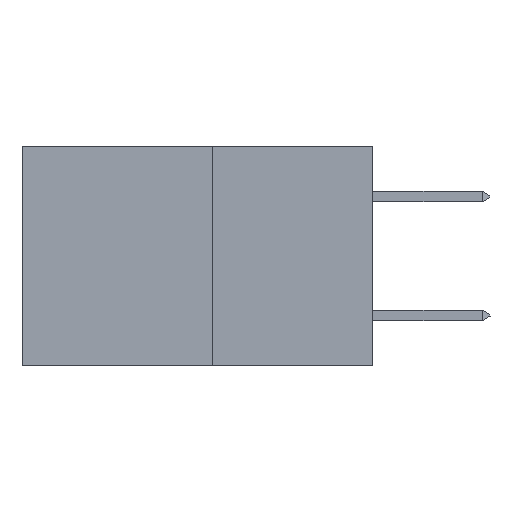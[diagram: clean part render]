
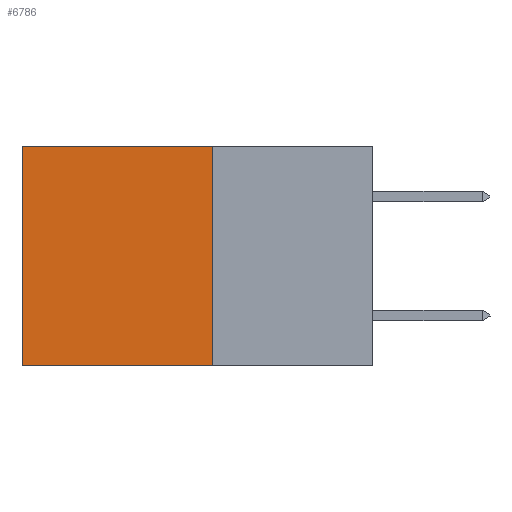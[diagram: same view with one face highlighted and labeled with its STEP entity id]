
A CAD part, left-side view. The second image highlights one B-rep face of the part: STEP entity #6786.
In plain terms, the highlighted planar face has unit normal (-1, 0, 0).
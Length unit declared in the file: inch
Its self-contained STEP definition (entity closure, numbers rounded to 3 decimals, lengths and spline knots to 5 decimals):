
#209 = CARTESIAN_POINT ( 'NONE',  ( 0.277, 0.27, -0.37 ) ) ;
#285 = EDGE_CURVE ( 'NONE', #6105, #10315, #3829, .T. ) ;
#513 = CARTESIAN_POINT ( 'NONE',  ( 0.277, 0.59, 0. ) ) ;
#526 = EDGE_CURVE ( 'NONE', #11175, #8962, #9156, .T. ) ;
#1285 = ORIENTED_EDGE ( 'NONE', *, *, #2825, .T. ) ;
#1349 = ORIENTED_EDGE ( 'NONE', *, *, #285, .F. ) ;
#1584 = ORIENTED_EDGE ( 'NONE', *, *, #9762, .F. ) ;
#1622 = ORIENTED_EDGE ( 'NONE', *, *, #526, .T. ) ;
#1782 = DIRECTION ( 'NONE',  ( 0., 1., 0. ) ) ;
#2012 = VECTOR ( 'NONE', #3813, 39.37008 ) ;
#2354 = DIRECTION ( 'NONE',  ( 1., 0., 0. ) ) ;
#2708 = LINE ( 'NONE', #10330, #4684 ) ;
#2825 = EDGE_CURVE ( 'NONE', #8962, #10315, #4602, .T. ) ;
#2846 = CARTESIAN_POINT ( 'NONE',  ( 0.277, 0.27, 0. ) ) ;
#3629 = CARTESIAN_POINT ( 'NONE',  ( 0.277, 0.27, -0.37 ) ) ;
#3813 = DIRECTION ( 'NONE',  ( 0., 0., -1. ) ) ;
#3829 = LINE ( 'NONE', #5829, #10725 ) ;
#3941 = FACE_OUTER_BOUND ( 'NONE', #11182, .T. ) ;
#4111 = VECTOR ( 'NONE', #9758, 39.37008 ) ;
#4602 = LINE ( 'NONE', #11454, #2012 ) ;
#4684 = VECTOR ( 'NONE', #6207, 39.37008 ) ;
#5293 = CARTESIAN_POINT ( 'NONE',  ( 0.277, 0.27, 0. ) ) ;
#5829 = CARTESIAN_POINT ( 'NONE',  ( 0.277, 0.27, -0.37 ) ) ;
#6105 = VERTEX_POINT ( 'NONE', #3629 ) ;
#6207 = DIRECTION ( 'NONE',  ( 0., 0., -1. ) ) ;
#6549 = AXIS2_PLACEMENT_3D ( 'NONE', #209, #2354, #8776 ) ;
#6786 = ADVANCED_FACE ( 'NONE', ( #3941 ), #7928, .F. ) ;
#7928 = PLANE ( 'NONE',  #6549 ) ;
#8776 = DIRECTION ( 'NONE',  ( 0., 0., -1. ) ) ;
#8962 = VERTEX_POINT ( 'NONE', #513 ) ;
#9156 = LINE ( 'NONE', #5293, #4111 ) ;
#9226 = CARTESIAN_POINT ( 'NONE',  ( 0.277, 0.59, -0.37 ) ) ;
#9758 = DIRECTION ( 'NONE',  ( 0., 1., 0. ) ) ;
#9762 = EDGE_CURVE ( 'NONE', #11175, #6105, #2708, .T. ) ;
#10315 = VERTEX_POINT ( 'NONE', #9226 ) ;
#10330 = CARTESIAN_POINT ( 'NONE',  ( 0.277, 0.27, -0.37 ) ) ;
#10725 = VECTOR ( 'NONE', #1782, 39.37008 ) ;
#11175 = VERTEX_POINT ( 'NONE', #2846 ) ;
#11182 = EDGE_LOOP ( 'NONE', ( #1285, #1349, #1584, #1622 ) ) ;
#11454 = CARTESIAN_POINT ( 'NONE',  ( 0.277, 0.59, -0.37 ) ) ;
